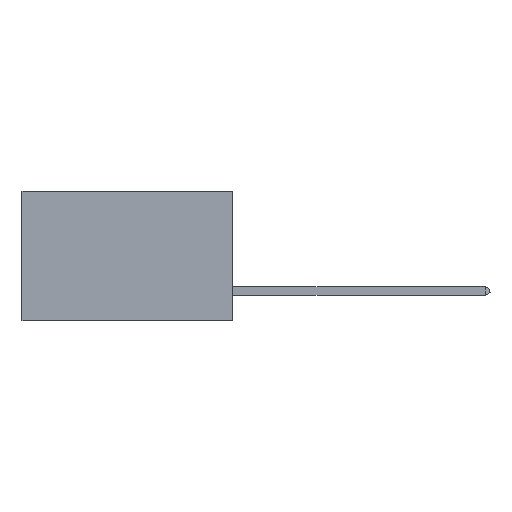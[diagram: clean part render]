
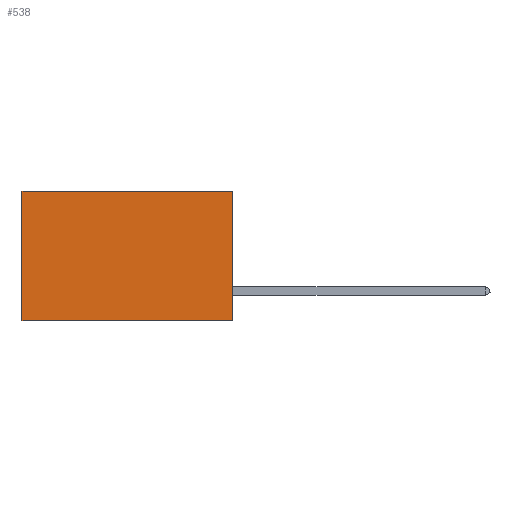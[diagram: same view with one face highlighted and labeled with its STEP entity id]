
A CAD part, left-side view. The second image highlights one B-rep face of the part: STEP entity #538.
In plain terms, the highlighted planar face has unit normal (-1, 0, 0).
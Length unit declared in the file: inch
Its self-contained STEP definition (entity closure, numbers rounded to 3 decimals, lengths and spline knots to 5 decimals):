
#46 = CARTESIAN_POINT ( 'NONE',  ( 0.2875, 0., 0. ) ) ;
#298 = VECTOR ( 'NONE', #13807, 39.37008 ) ;
#538 = ADVANCED_FACE ( 'NONE', ( #3975 ), #14262, .F. ) ;
#2221 = LINE ( 'NONE', #46, #298 ) ;
#2251 = VERTEX_POINT ( 'NONE', #12051 ) ;
#2552 = CARTESIAN_POINT ( 'NONE',  ( 0.2875, 0., -0.37 ) ) ;
#2623 = LINE ( 'NONE', #13513, #5507 ) ;
#2702 = LINE ( 'NONE', #4319, #6341 ) ;
#3107 = CARTESIAN_POINT ( 'NONE',  ( 0.2875, 0.6, -0.37 ) ) ;
#3409 = CARTESIAN_POINT ( 'NONE',  ( 0.2875, 0., 0. ) ) ;
#3975 = FACE_OUTER_BOUND ( 'NONE', #10284, .T. ) ;
#4194 = EDGE_CURVE ( 'NONE', #12899, #12969, #10025, .T. ) ;
#4319 = CARTESIAN_POINT ( 'NONE',  ( 0.2875, 0., 0. ) ) ;
#5335 = ORIENTED_EDGE ( 'NONE', *, *, #11465, .T. ) ;
#5452 = ORIENTED_EDGE ( 'NONE', *, *, #4194, .F. ) ;
#5507 = VECTOR ( 'NONE', #8397, 39.37008 ) ;
#5627 = ORIENTED_EDGE ( 'NONE', *, *, #5979, .T. ) ;
#5979 = EDGE_CURVE ( 'NONE', #6258, #2251, #2221, .T. ) ;
#6258 = VERTEX_POINT ( 'NONE', #3409 ) ;
#6341 = VECTOR ( 'NONE', #10465, 39.37008 ) ;
#6714 = VECTOR ( 'NONE', #15902, 39.37008 ) ;
#8163 = DIRECTION ( 'NONE',  ( 1., 0., 0. ) ) ;
#8397 = DIRECTION ( 'NONE',  ( 0., 0., -1. ) ) ;
#8642 = EDGE_CURVE ( 'NONE', #6258, #12899, #2702, .T. ) ;
#9337 = CARTESIAN_POINT ( 'NONE',  ( 0.2875, 0., 0. ) ) ;
#9442 = DIRECTION ( 'NONE',  ( 0., 0., -1. ) ) ;
#10025 = LINE ( 'NONE', #2552, #6714 ) ;
#10284 = EDGE_LOOP ( 'NONE', ( #5335, #5452, #13066, #5627 ) ) ;
#10465 = DIRECTION ( 'NONE',  ( 0., 0., -1. ) ) ;
#10634 = AXIS2_PLACEMENT_3D ( 'NONE', #9337, #8163, #9442 ) ;
#11465 = EDGE_CURVE ( 'NONE', #2251, #12969, #2623, .T. ) ;
#11582 = CARTESIAN_POINT ( 'NONE',  ( 0.2875, 0., -0.37 ) ) ;
#12051 = CARTESIAN_POINT ( 'NONE',  ( 0.2875, 0.6, 0. ) ) ;
#12899 = VERTEX_POINT ( 'NONE', #11582 ) ;
#12969 = VERTEX_POINT ( 'NONE', #3107 ) ;
#13066 = ORIENTED_EDGE ( 'NONE', *, *, #8642, .F. ) ;
#13513 = CARTESIAN_POINT ( 'NONE',  ( 0.2875, 0.6, 0. ) ) ;
#13807 = DIRECTION ( 'NONE',  ( 0., 1., 0. ) ) ;
#14262 = PLANE ( 'NONE',  #10634 ) ;
#15902 = DIRECTION ( 'NONE',  ( 0., 1., 0. ) ) ;
